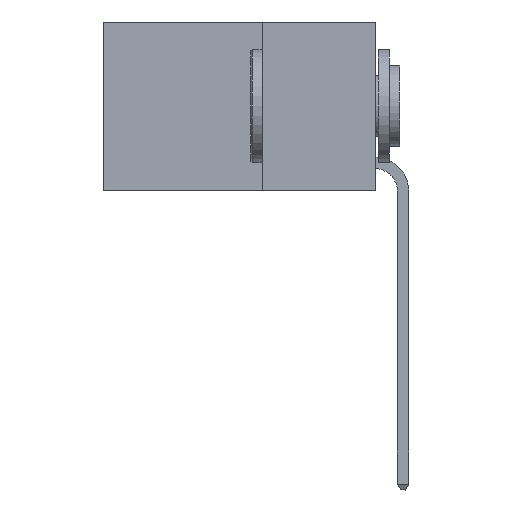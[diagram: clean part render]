
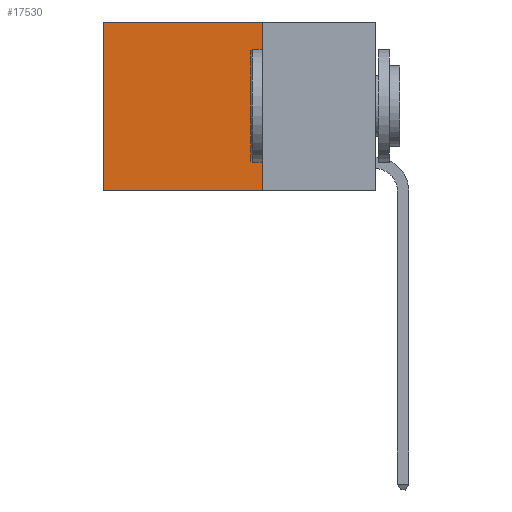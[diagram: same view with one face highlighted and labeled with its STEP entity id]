
A CAD part, left-side view. The second image highlights one B-rep face of the part: STEP entity #17530.
In plain terms, the highlighted planar face has unit normal (-1, 0, 0).
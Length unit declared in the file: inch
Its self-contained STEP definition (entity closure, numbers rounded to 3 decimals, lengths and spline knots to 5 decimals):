
#277 = CARTESIAN_POINT ( 'NONE',  ( 0.2625, 0.25, -0.37 ) ) ;
#353 = FACE_OUTER_BOUND ( 'NONE', #15813, .T. ) ;
#1291 = CARTESIAN_POINT ( 'NONE',  ( 0.2625, 0.25, 0. ) ) ;
#1696 = VERTEX_POINT ( 'NONE', #13425 ) ;
#1877 = DIRECTION ( 'NONE',  ( 0., 0., -1. ) ) ;
#2145 = LINE ( 'NONE', #277, #20269 ) ;
#4144 = CARTESIAN_POINT ( 'NONE',  ( 0.2625, 0.25, 0. ) ) ;
#4562 = CARTESIAN_POINT ( 'NONE',  ( 0.2625, 0.6, -0.37 ) ) ;
#4974 = VECTOR ( 'NONE', #8614, 39.37008 ) ;
#5236 = AXIS2_PLACEMENT_3D ( 'NONE', #4144, #16032, #1877 ) ;
#5367 = ORIENTED_EDGE ( 'NONE', *, *, #21407, .T. ) ;
#5752 = CARTESIAN_POINT ( 'NONE',  ( 0.2625, 0.25, -0.37 ) ) ;
#6159 = LINE ( 'NONE', #1291, #11702 ) ;
#6242 = CARTESIAN_POINT ( 'NONE',  ( 0.2625, 0.25, 0. ) ) ;
#8614 = DIRECTION ( 'NONE',  ( 0., 0., -1. ) ) ;
#11702 = VECTOR ( 'NONE', #24950, 39.37008 ) ;
#12016 = VECTOR ( 'NONE', #25039, 39.37008 ) ;
#12089 = DIRECTION ( 'NONE',  ( 0., 1., 0. ) ) ;
#12786 = CARTESIAN_POINT ( 'NONE',  ( 0.2625, 0.6, 0. ) ) ;
#13255 = CARTESIAN_POINT ( 'NONE',  ( 0.2625, 0.6, 0. ) ) ;
#13425 = CARTESIAN_POINT ( 'NONE',  ( 0.2625, 0.25, 0. ) ) ;
#13646 = PLANE ( 'NONE',  #5236 ) ;
#14878 = VERTEX_POINT ( 'NONE', #5752 ) ;
#15717 = VERTEX_POINT ( 'NONE', #4562 ) ;
#15813 = EDGE_LOOP ( 'NONE', ( #5367, #26954, #22704, #20481 ) ) ;
#16032 = DIRECTION ( 'NONE',  ( 1., 0., 0. ) ) ;
#17530 = ADVANCED_FACE ( 'NONE', ( #353 ), #13646, .F. ) ;
#18301 = LINE ( 'NONE', #13255, #12016 ) ;
#20269 = VECTOR ( 'NONE', #12089, 39.37008 ) ;
#20481 = ORIENTED_EDGE ( 'NONE', *, *, #29543, .T. ) ;
#21407 = EDGE_CURVE ( 'NONE', #25332, #15717, #18301, .T. ) ;
#21416 = EDGE_CURVE ( 'NONE', #1696, #14878, #30160, .T. ) ;
#22704 = ORIENTED_EDGE ( 'NONE', *, *, #21416, .F. ) ;
#24950 = DIRECTION ( 'NONE',  ( 0., 1., 0. ) ) ;
#25039 = DIRECTION ( 'NONE',  ( 0., 0., -1. ) ) ;
#25332 = VERTEX_POINT ( 'NONE', #12786 ) ;
#26954 = ORIENTED_EDGE ( 'NONE', *, *, #28606, .F. ) ;
#28606 = EDGE_CURVE ( 'NONE', #14878, #15717, #2145, .T. ) ;
#29543 = EDGE_CURVE ( 'NONE', #1696, #25332, #6159, .T. ) ;
#30160 = LINE ( 'NONE', #6242, #4974 ) ;
